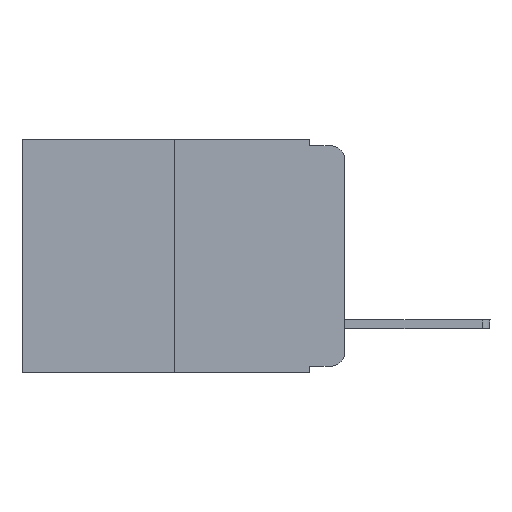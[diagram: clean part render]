
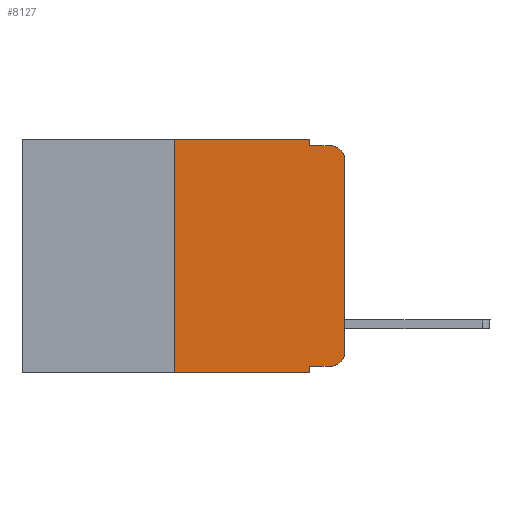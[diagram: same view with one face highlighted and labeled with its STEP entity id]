
A CAD part, left-side view. The second image highlights one B-rep face of the part: STEP entity #8127.
In plain terms, the highlighted planar face has unit normal (-1, 0, 0).
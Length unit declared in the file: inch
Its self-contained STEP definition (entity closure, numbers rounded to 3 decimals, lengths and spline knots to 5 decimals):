
#108 = CARTESIAN_POINT ( 'NONE',  ( 0., 0.051, -0.01 ) ) ;
#179 = VERTEX_POINT ( 'NONE', #13989 ) ;
#403 = LINE ( 'NONE', #12749, #16952 ) ;
#921 = AXIS2_PLACEMENT_3D ( 'NONE', #18335, #9209, #7699 ) ;
#1207 = ORIENTED_EDGE ( 'NONE', *, *, #2287, .F. ) ;
#1378 = VERTEX_POINT ( 'NONE', #2303 ) ;
#1883 = DIRECTION ( 'NONE',  ( 0., 0., -1. ) ) ;
#1895 = CARTESIAN_POINT ( 'NONE',  ( 0., 0.051, 0. ) ) ;
#1925 = VECTOR ( 'NONE', #17029, 39.37008 ) ;
#1999 = LINE ( 'NONE', #3072, #17433 ) ;
#2142 = CARTESIAN_POINT ( 'NONE',  ( 0., 0.051, 0. ) ) ;
#2250 = DIRECTION ( 'NONE',  ( 0., -1., 0. ) ) ;
#2287 = EDGE_CURVE ( 'NONE', #11233, #8162, #14916, .T. ) ;
#2303 = CARTESIAN_POINT ( 'NONE',  ( 0., 0., -0.313 ) ) ;
#2534 = LINE ( 'NONE', #16853, #14320 ) ;
#2570 = LINE ( 'NONE', #8192, #1925 ) ;
#2861 = CARTESIAN_POINT ( 'NONE',  ( 0., 0.25, -0.343 ) ) ;
#2938 = CIRCLE ( 'NONE', #15388, 0.02 ) ;
#3072 = CARTESIAN_POINT ( 'NONE',  ( 0., 0.051, 0. ) ) ;
#3325 = DIRECTION ( 'NONE',  ( 0., 0., -1. ) ) ;
#4220 = ORIENTED_EDGE ( 'NONE', *, *, #5641, .T. ) ;
#4302 = AXIS2_PLACEMENT_3D ( 'NONE', #8913, #4485, #6053 ) ;
#4485 = DIRECTION ( 'NONE',  ( 1., 0., 0. ) ) ;
#4906 = CARTESIAN_POINT ( 'NONE',  ( 0., 0., -0.03 ) ) ;
#4912 = VERTEX_POINT ( 'NONE', #12771 ) ;
#5100 = EDGE_CURVE ( 'NONE', #7216, #12462, #403, .T. ) ;
#5270 = LINE ( 'NONE', #14099, #17785 ) ;
#5293 = ORIENTED_EDGE ( 'NONE', *, *, #13721, .F. ) ;
#5479 = DIRECTION ( 'NONE',  ( 0., -1., 0. ) ) ;
#5620 = DIRECTION ( 'NONE',  ( 0., -1., 0. ) ) ;
#5641 = EDGE_CURVE ( 'NONE', #179, #14188, #8064, .T. ) ;
#5845 = EDGE_CURVE ( 'NONE', #8162, #10025, #8963, .T. ) ;
#6018 = CARTESIAN_POINT ( 'NONE',  ( 0., 0.02, -0.03 ) ) ;
#6053 = DIRECTION ( 'NONE',  ( 0., 0., -1. ) ) ;
#6602 = EDGE_LOOP ( 'NONE', ( #18187, #14940, #11267, #1207, #5293, #8093, #15524, #15375, #4220, #11530 ) ) ;
#7216 = VERTEX_POINT ( 'NONE', #2861 ) ;
#7699 = DIRECTION ( 'NONE',  ( 0., 0., -1. ) ) ;
#8064 = LINE ( 'NONE', #18312, #18515 ) ;
#8093 = ORIENTED_EDGE ( 'NONE', *, *, #18349, .F. ) ;
#8127 = ADVANCED_FACE ( 'NONE', ( #10123 ), #11736, .F. ) ;
#8162 = VERTEX_POINT ( 'NONE', #108 ) ;
#8192 = CARTESIAN_POINT ( 'NONE',  ( 0., 0.25, 0. ) ) ;
#8252 = DIRECTION ( 'NONE',  ( 0., 0., 1. ) ) ;
#8913 = CARTESIAN_POINT ( 'NONE',  ( 0., 0.473, 0. ) ) ;
#8963 = LINE ( 'NONE', #17240, #14183 ) ;
#9022 = DIRECTION ( 'NONE',  ( -1., 0., 0. ) ) ;
#9209 = DIRECTION ( 'NONE',  ( -1., 0., 0. ) ) ;
#10025 = VERTEX_POINT ( 'NONE', #11729 ) ;
#10123 = FACE_OUTER_BOUND ( 'NONE', #6602, .T. ) ;
#10147 = VERTEX_POINT ( 'NONE', #4906 ) ;
#10231 = CARTESIAN_POINT ( 'NONE',  ( 0., 0.02, -0.333 ) ) ;
#10836 = EDGE_CURVE ( 'NONE', #14188, #1378, #12966, .T. ) ;
#10984 = DIRECTION ( 'NONE',  ( 0., -1., 0. ) ) ;
#11233 = VERTEX_POINT ( 'NONE', #2142 ) ;
#11267 = ORIENTED_EDGE ( 'NONE', *, *, #5845, .F. ) ;
#11530 = ORIENTED_EDGE ( 'NONE', *, *, #10836, .T. ) ;
#11729 = CARTESIAN_POINT ( 'NONE',  ( 0., 0.02, -0.01 ) ) ;
#11736 = PLANE ( 'NONE',  #4302 ) ;
#11783 = EDGE_CURVE ( 'NONE', #10147, #10025, #2938, .T. ) ;
#12462 = VERTEX_POINT ( 'NONE', #14782 ) ;
#12749 = CARTESIAN_POINT ( 'NONE',  ( 0., 0.473, -0.343 ) ) ;
#12771 = CARTESIAN_POINT ( 'NONE',  ( 0., 0.25, 0. ) ) ;
#12932 = EDGE_CURVE ( 'NONE', #179, #12462, #1999, .T. ) ;
#12966 = CIRCLE ( 'NONE', #921, 0.02 ) ;
#13175 = DIRECTION ( 'NONE',  ( 0., 0., -1. ) ) ;
#13721 = EDGE_CURVE ( 'NONE', #4912, #11233, #2534, .T. ) ;
#13989 = CARTESIAN_POINT ( 'NONE',  ( 0., 0.051, -0.333 ) ) ;
#14099 = CARTESIAN_POINT ( 'NONE',  ( 0., 0., 0. ) ) ;
#14183 = VECTOR ( 'NONE', #5620, 39.37008 ) ;
#14188 = VERTEX_POINT ( 'NONE', #10231 ) ;
#14320 = VECTOR ( 'NONE', #2250, 39.37008 ) ;
#14782 = CARTESIAN_POINT ( 'NONE',  ( 0., 0.051, -0.343 ) ) ;
#14916 = LINE ( 'NONE', #1895, #18768 ) ;
#14940 = ORIENTED_EDGE ( 'NONE', *, *, #11783, .T. ) ;
#15375 = ORIENTED_EDGE ( 'NONE', *, *, #12932, .F. ) ;
#15388 = AXIS2_PLACEMENT_3D ( 'NONE', #6018, #9022, #1883 ) ;
#15524 = ORIENTED_EDGE ( 'NONE', *, *, #5100, .T. ) ;
#16853 = CARTESIAN_POINT ( 'NONE',  ( 0., 0.473, 0. ) ) ;
#16952 = VECTOR ( 'NONE', #5479, 39.37008 ) ;
#17029 = DIRECTION ( 'NONE',  ( 0., 0., 1. ) ) ;
#17240 = CARTESIAN_POINT ( 'NONE',  ( 0., 0.051, -0.01 ) ) ;
#17433 = VECTOR ( 'NONE', #13175, 39.37008 ) ;
#17785 = VECTOR ( 'NONE', #8252, 39.37008 ) ;
#18187 = ORIENTED_EDGE ( 'NONE', *, *, #18344, .T. ) ;
#18312 = CARTESIAN_POINT ( 'NONE',  ( 0., 0.051, -0.333 ) ) ;
#18335 = CARTESIAN_POINT ( 'NONE',  ( 0., 0.02, -0.313 ) ) ;
#18344 = EDGE_CURVE ( 'NONE', #1378, #10147, #5270, .T. ) ;
#18349 = EDGE_CURVE ( 'NONE', #7216, #4912, #2570, .T. ) ;
#18515 = VECTOR ( 'NONE', #10984, 39.37008 ) ;
#18768 = VECTOR ( 'NONE', #3325, 39.37008 ) ;
